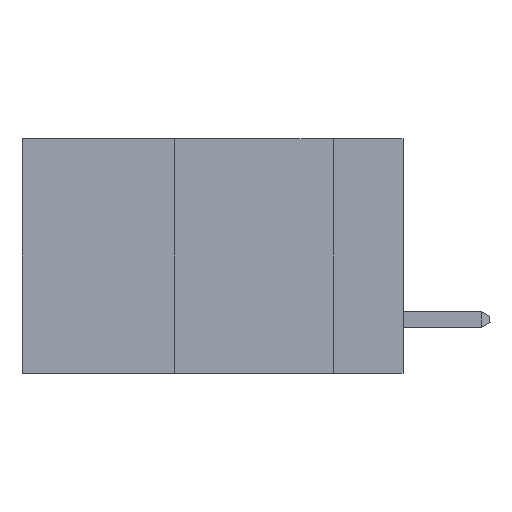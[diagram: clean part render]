
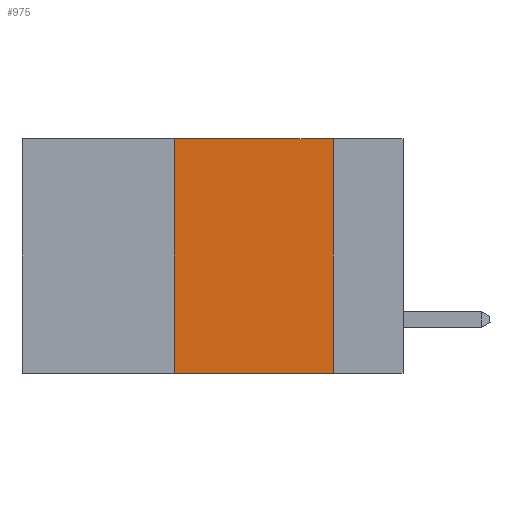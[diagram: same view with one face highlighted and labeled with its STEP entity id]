
A CAD part, left-side view. The second image highlights one B-rep face of the part: STEP entity #975.
In plain terms, the highlighted planar face has unit normal (-1, 0, 0).
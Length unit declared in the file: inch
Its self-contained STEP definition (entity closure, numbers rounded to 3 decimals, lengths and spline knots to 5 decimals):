
#634 = VERTEX_POINT ( 'NONE', #10349 ) ;
#636 = VECTOR ( 'NONE', #2146, 39.37008 ) ;
#975 = ADVANCED_FACE ( 'NONE', ( #13275 ), #6338, .F. ) ;
#1128 = ORIENTED_EDGE ( 'NONE', *, *, #14961, .F. ) ;
#1256 = CARTESIAN_POINT ( 'NONE',  ( 0., 0.36, 0. ) ) ;
#1572 = VERTEX_POINT ( 'NONE', #2688 ) ;
#1587 = DIRECTION ( 'NONE',  ( 1., 0., 0. ) ) ;
#1617 = CARTESIAN_POINT ( 'NONE',  ( 0., 0.6, -0.37 ) ) ;
#1670 = DIRECTION ( 'NONE',  ( 0., -1., 0. ) ) ;
#1709 = LINE ( 'NONE', #11393, #636 ) ;
#1807 = EDGE_CURVE ( 'NONE', #6398, #634, #2111, .T. ) ;
#1903 = DIRECTION ( 'NONE',  ( 0., -1., 0. ) ) ;
#2111 = LINE ( 'NONE', #14832, #4142 ) ;
#2146 = DIRECTION ( 'NONE',  ( 0., 0., -1. ) ) ;
#2316 = DIRECTION ( 'NONE',  ( 0., 0., 1. ) ) ;
#2688 = CARTESIAN_POINT ( 'NONE',  ( 0., 0.11, -0.37 ) ) ;
#3151 = VECTOR ( 'NONE', #2316, 39.37008 ) ;
#4142 = VECTOR ( 'NONE', #1903, 39.37008 ) ;
#5266 = EDGE_CURVE ( 'NONE', #634, #1572, #1709, .T. ) ;
#6338 = PLANE ( 'NONE',  #10361 ) ;
#6398 = VERTEX_POINT ( 'NONE', #14040 ) ;
#6407 = VECTOR ( 'NONE', #1670, 39.37008 ) ;
#6585 = ORIENTED_EDGE ( 'NONE', *, *, #7269, .T. ) ;
#7269 = EDGE_CURVE ( 'NONE', #10526, #1572, #9107, .T. ) ;
#7511 = EDGE_LOOP ( 'NONE', ( #11480, #10277, #1128, #6585 ) ) ;
#8377 = CARTESIAN_POINT ( 'NONE',  ( 0., 0.36, -0.37 ) ) ;
#8513 = CARTESIAN_POINT ( 'NONE',  ( 0., 0.6, 0. ) ) ;
#9107 = LINE ( 'NONE', #1617, #6407 ) ;
#9727 = DIRECTION ( 'NONE',  ( 0., 0., -1. ) ) ;
#10277 = ORIENTED_EDGE ( 'NONE', *, *, #1807, .F. ) ;
#10349 = CARTESIAN_POINT ( 'NONE',  ( 0., 0.11, 0. ) ) ;
#10361 = AXIS2_PLACEMENT_3D ( 'NONE', #8513, #1587, #9727 ) ;
#10526 = VERTEX_POINT ( 'NONE', #8377 ) ;
#11393 = CARTESIAN_POINT ( 'NONE',  ( 0., 0.11, 0. ) ) ;
#11480 = ORIENTED_EDGE ( 'NONE', *, *, #5266, .F. ) ;
#11859 = LINE ( 'NONE', #1256, #3151 ) ;
#13275 = FACE_OUTER_BOUND ( 'NONE', #7511, .T. ) ;
#14040 = CARTESIAN_POINT ( 'NONE',  ( 0., 0.36, 0. ) ) ;
#14832 = CARTESIAN_POINT ( 'NONE',  ( 0., 0.6, 0. ) ) ;
#14961 = EDGE_CURVE ( 'NONE', #10526, #6398, #11859, .T. ) ;
